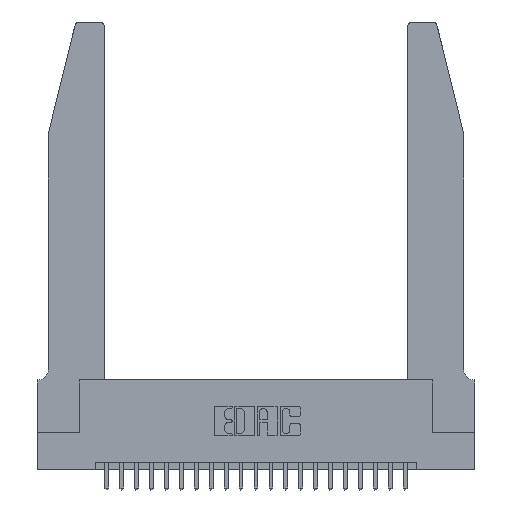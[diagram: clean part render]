
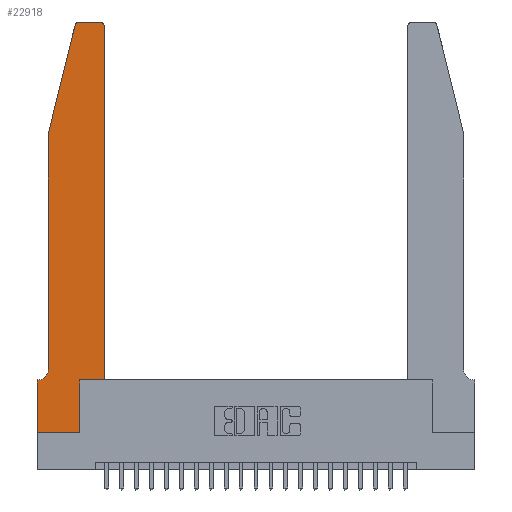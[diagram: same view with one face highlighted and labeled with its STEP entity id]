
A CAD part, top view. The second image highlights one B-rep face of the part: STEP entity #22918.
In plain terms, the highlighted planar face has unit normal (0, 0, 1).
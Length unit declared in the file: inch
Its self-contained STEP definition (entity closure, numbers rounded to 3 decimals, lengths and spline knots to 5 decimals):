
#471 = LINE ( 'NONE', #4281, #19753 ) ;
#1038 = DIRECTION ( 'NONE',  ( -1., 0., 0. ) ) ;
#1086 = VECTOR ( 'NONE', #23854, 39.37008 ) ;
#1204 = VECTOR ( 'NONE', #21903, 39.37008 ) ;
#1248 = EDGE_CURVE ( 'NONE', #1481, #22786, #471, .T. ) ;
#1299 = CARTESIAN_POINT ( 'NONE',  ( 0.0755, 2., 0.37 ) ) ;
#1429 = DIRECTION ( 'NONE',  ( 1., 0., 0. ) ) ;
#1481 = VERTEX_POINT ( 'NONE', #6994 ) ;
#1819 = DIRECTION ( 'NONE',  ( 1., 0., 0. ) ) ;
#1891 = EDGE_CURVE ( 'NONE', #11632, #19536, #3139, .T. ) ;
#2219 = VECTOR ( 'NONE', #10504, 39.37008 ) ;
#2279 = VERTEX_POINT ( 'NONE', #8653 ) ;
#2448 = DIRECTION ( 'NONE',  ( 0., 0., -1. ) ) ;
#2814 = AXIS2_PLACEMENT_3D ( 'NONE', #13674, #2448, #15524 ) ;
#3139 = LINE ( 'NONE', #1299, #7005 ) ;
#3159 = ORIENTED_EDGE ( 'NONE', *, *, #1248, .T. ) ;
#3364 = ORIENTED_EDGE ( 'NONE', *, *, #17831, .T. ) ;
#3489 = CARTESIAN_POINT ( 'NONE',  ( 0.4505, 0.35, 0.37 ) ) ;
#3719 = CARTESIAN_POINT ( 'NONE',  ( 0., 0.35, 0.37 ) ) ;
#4034 = ORIENTED_EDGE ( 'NONE', *, *, #9789, .T. ) ;
#4281 = CARTESIAN_POINT ( 'NONE',  ( 0.4505, 0.35, 0.37 ) ) ;
#4409 = CARTESIAN_POINT ( 'NONE',  ( 0.4205, 2.75, 0.37 ) ) ;
#5412 = DIRECTION ( 'NONE',  ( 0., 1., 0. ) ) ;
#6301 = VECTOR ( 'NONE', #18497, 39.37008 ) ;
#6402 = CARTESIAN_POINT ( 'NONE',  ( 0.2865, 0., 0.37 ) ) ;
#6670 = CARTESIAN_POINT ( 'NONE',  ( 0.4505, 0.35, 0.37 ) ) ;
#6994 = CARTESIAN_POINT ( 'NONE',  ( 0.2865, 0.35, 0.37 ) ) ;
#7005 = VECTOR ( 'NONE', #12543, 39.37008 ) ;
#7473 = LINE ( 'NONE', #16646, #6301 ) ;
#7775 = EDGE_CURVE ( 'NONE', #14603, #10210, #17334, .T. ) ;
#8044 = CARTESIAN_POINT ( 'NONE',  ( 0., 0., 0.37 ) ) ;
#8086 = ORIENTED_EDGE ( 'NONE', *, *, #11789, .T. ) ;
#8148 = VERTEX_POINT ( 'NONE', #20706 ) ;
#8220 = CARTESIAN_POINT ( 'NONE',  ( 0.0755, 2., 0.37 ) ) ;
#8653 = CARTESIAN_POINT ( 'NONE',  ( 0.284, 2.75, 0.37 ) ) ;
#8880 = PLANE ( 'NONE',  #11124 ) ;
#9786 = DIRECTION ( 'NONE',  ( 1., 0., 0. ) ) ;
#9789 = EDGE_CURVE ( 'NONE', #8148, #23247, #14097, .T. ) ;
#9894 = EDGE_LOOP ( 'NONE', ( #11894, #18799, #3364, #10991, #23357, #8086, #14001, #12266, #11099, #3159, #14537, #4034 ) ) ;
#10210 = VERTEX_POINT ( 'NONE', #6402 ) ;
#10504 = DIRECTION ( 'NONE',  ( -1., 0., 0. ) ) ;
#10595 = CARTESIAN_POINT ( 'NONE',  ( 0., 0., 0.37 ) ) ;
#10755 = CARTESIAN_POINT ( 'NONE',  ( 0., 0.35, 0.37 ) ) ;
#10800 = VERTEX_POINT ( 'NONE', #12627 ) ;
#10865 = EDGE_CURVE ( 'NONE', #17236, #14603, #20883, .T. ) ;
#10991 = ORIENTED_EDGE ( 'NONE', *, *, #1891, .T. ) ;
#11099 = ORIENTED_EDGE ( 'NONE', *, *, #18736, .T. ) ;
#11124 = AXIS2_PLACEMENT_3D ( 'NONE', #10755, #23590, #12596 ) ;
#11184 = EDGE_CURVE ( 'NONE', #23247, #2279, #14530, .T. ) ;
#11530 = CIRCLE ( 'NONE', #2814, 0.07 ) ;
#11582 = FACE_OUTER_BOUND ( 'NONE', #9894, .T. ) ;
#11632 = VERTEX_POINT ( 'NONE', #8220 ) ;
#11789 = EDGE_CURVE ( 'NONE', #17520, #17236, #20839, .T. ) ;
#11894 = ORIENTED_EDGE ( 'NONE', *, *, #11184, .T. ) ;
#12266 = ORIENTED_EDGE ( 'NONE', *, *, #7775, .T. ) ;
#12543 = DIRECTION ( 'NONE',  ( 0., -1., 0. ) ) ;
#12596 = DIRECTION ( 'NONE',  ( 1., 0., 0. ) ) ;
#12627 = CARTESIAN_POINT ( 'NONE',  ( 0.25487, 2.72718, 0.37 ) ) ;
#12646 = AXIS2_PLACEMENT_3D ( 'NONE', #23666, #12672, #1429 ) ;
#12672 = DIRECTION ( 'NONE',  ( 0., 0., 1. ) ) ;
#13038 = DIRECTION ( 'NONE',  ( 0., 0., 1. ) ) ;
#13287 = LINE ( 'NONE', #3489, #22466 ) ;
#13479 = EDGE_CURVE ( 'NONE', #19536, #17520, #11530, .T. ) ;
#13674 = CARTESIAN_POINT ( 'NONE',  ( 0.0055, 0.42, 0.37 ) ) ;
#14001 = ORIENTED_EDGE ( 'NONE', *, *, #10865, .T. ) ;
#14097 = CIRCLE ( 'NONE', #12646, 0.03 ) ;
#14530 = LINE ( 'NONE', #15931, #23720 ) ;
#14537 = ORIENTED_EDGE ( 'NONE', *, *, #16730, .T. ) ;
#14603 = VERTEX_POINT ( 'NONE', #8044 ) ;
#15524 = DIRECTION ( 'NONE',  ( -1., 0., 0. ) ) ;
#15931 = CARTESIAN_POINT ( 'NONE',  ( 0.2605, 2.75, 0.37 ) ) ;
#16130 = LINE ( 'NONE', #20089, #1204 ) ;
#16493 = CARTESIAN_POINT ( 'NONE',  ( 0., 0., 0.37 ) ) ;
#16593 = CARTESIAN_POINT ( 'NONE',  ( 0.0755, 0.42, 0.37 ) ) ;
#16646 = CARTESIAN_POINT ( 'NONE',  ( 0.0755, 2., 0.37 ) ) ;
#16730 = EDGE_CURVE ( 'NONE', #22786, #8148, #13287, .T. ) ;
#16747 = VECTOR ( 'NONE', #19774, 39.37008 ) ;
#17186 = EDGE_CURVE ( 'NONE', #2279, #10800, #19069, .T. ) ;
#17236 = VERTEX_POINT ( 'NONE', #3719 ) ;
#17334 = LINE ( 'NONE', #10595, #16747 ) ;
#17520 = VERTEX_POINT ( 'NONE', #23083 ) ;
#17831 = EDGE_CURVE ( 'NONE', #10800, #11632, #7473, .T. ) ;
#18497 = DIRECTION ( 'NONE',  ( -0.239, -0.971, 0. ) ) ;
#18736 = EDGE_CURVE ( 'NONE', #10210, #1481, #16130, .T. ) ;
#18799 = ORIENTED_EDGE ( 'NONE', *, *, #17186, .T. ) ;
#19069 = CIRCLE ( 'NONE', #20617, 0.03 ) ;
#19536 = VERTEX_POINT ( 'NONE', #16593 ) ;
#19753 = VECTOR ( 'NONE', #9786, 39.37008 ) ;
#19774 = DIRECTION ( 'NONE',  ( 1., 0., 0. ) ) ;
#20089 = CARTESIAN_POINT ( 'NONE',  ( 0.2865, 0.35, 0.37 ) ) ;
#20617 = AXIS2_PLACEMENT_3D ( 'NONE', #24030, #13038, #1819 ) ;
#20706 = CARTESIAN_POINT ( 'NONE',  ( 0.4505, 2.72, 0.37 ) ) ;
#20839 = LINE ( 'NONE', #23352, #2219 ) ;
#20883 = LINE ( 'NONE', #16493, #1086 ) ;
#21903 = DIRECTION ( 'NONE',  ( 0., 1., 0. ) ) ;
#22466 = VECTOR ( 'NONE', #5412, 39.37008 ) ;
#22786 = VERTEX_POINT ( 'NONE', #6670 ) ;
#22918 = ADVANCED_FACE ( 'NONE', ( #11582 ), #8880, .T. ) ;
#23083 = CARTESIAN_POINT ( 'NONE',  ( 0.0055, 0.35, 0.37 ) ) ;
#23247 = VERTEX_POINT ( 'NONE', #4409 ) ;
#23352 = CARTESIAN_POINT ( 'NONE',  ( 0.0755, 0.35, 0.37 ) ) ;
#23357 = ORIENTED_EDGE ( 'NONE', *, *, #13479, .T. ) ;
#23590 = DIRECTION ( 'NONE',  ( 0., 0., 1. ) ) ;
#23666 = CARTESIAN_POINT ( 'NONE',  ( 0.4205, 2.72, 0.37 ) ) ;
#23720 = VECTOR ( 'NONE', #1038, 39.37008 ) ;
#23854 = DIRECTION ( 'NONE',  ( 0., -1., 0. ) ) ;
#24030 = CARTESIAN_POINT ( 'NONE',  ( 0.284, 2.72, 0.37 ) ) ;
